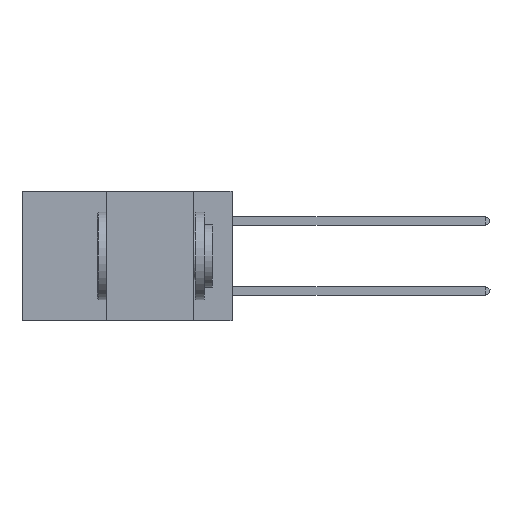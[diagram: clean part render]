
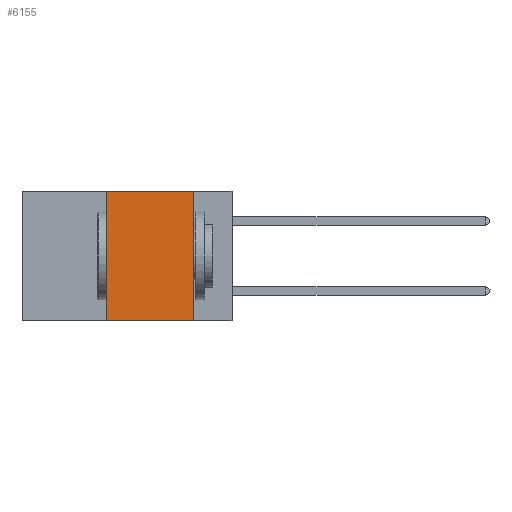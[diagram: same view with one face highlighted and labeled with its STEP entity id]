
A CAD part, left-side view. The second image highlights one B-rep face of the part: STEP entity #6155.
In plain terms, the highlighted planar face has unit normal (-1, 0, 0).
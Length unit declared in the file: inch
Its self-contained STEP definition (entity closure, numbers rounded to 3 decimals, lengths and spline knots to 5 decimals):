
#76 = VECTOR ( 'NONE', #8333, 39.37008 ) ;
#557 = DIRECTION ( 'NONE',  ( 0., 0., -1. ) ) ;
#728 = PLANE ( 'NONE',  #2168 ) ;
#819 = ORIENTED_EDGE ( 'NONE', *, *, #10191, .T. ) ;
#937 = ORIENTED_EDGE ( 'NONE', *, *, #7530, .F. ) ;
#1045 = VERTEX_POINT ( 'NONE', #1852 ) ;
#1852 = CARTESIAN_POINT ( 'NONE',  ( 0., 0.11, -0.37 ) ) ;
#2168 = AXIS2_PLACEMENT_3D ( 'NONE', #7407, #4162, #9220 ) ;
#2576 = CARTESIAN_POINT ( 'NONE',  ( 0., 0.36, 0. ) ) ;
#2775 = ORIENTED_EDGE ( 'NONE', *, *, #5032, .F. ) ;
#3537 = VECTOR ( 'NONE', #10254, 39.37008 ) ;
#3805 = VERTEX_POINT ( 'NONE', #9456 ) ;
#4162 = DIRECTION ( 'NONE',  ( 1., 0., 0. ) ) ;
#4769 = LINE ( 'NONE', #5936, #3537 ) ;
#5032 = EDGE_CURVE ( 'NONE', #3805, #1045, #9554, .T. ) ;
#5721 = LINE ( 'NONE', #2576, #6794 ) ;
#5936 = CARTESIAN_POINT ( 'NONE',  ( 0., 0.6, 0. ) ) ;
#6155 = ADVANCED_FACE ( 'NONE', ( #6179 ), #728, .F. ) ;
#6179 = FACE_OUTER_BOUND ( 'NONE', #7899, .T. ) ;
#6322 = CARTESIAN_POINT ( 'NONE',  ( 0., 0.36, 0. ) ) ;
#6646 = CARTESIAN_POINT ( 'NONE',  ( 0., 0.6, -0.37 ) ) ;
#6791 = VERTEX_POINT ( 'NONE', #9155 ) ;
#6794 = VECTOR ( 'NONE', #7733, 39.37008 ) ;
#7407 = CARTESIAN_POINT ( 'NONE',  ( 0., 0.6, 0. ) ) ;
#7530 = EDGE_CURVE ( 'NONE', #6791, #8830, #5721, .T. ) ;
#7684 = LINE ( 'NONE', #6646, #76 ) ;
#7733 = DIRECTION ( 'NONE',  ( 0., 0., 1. ) ) ;
#7734 = ORIENTED_EDGE ( 'NONE', *, *, #8209, .F. ) ;
#7899 = EDGE_LOOP ( 'NONE', ( #2775, #7734, #937, #819 ) ) ;
#8209 = EDGE_CURVE ( 'NONE', #8830, #3805, #4769, .T. ) ;
#8333 = DIRECTION ( 'NONE',  ( 0., -1., 0. ) ) ;
#8830 = VERTEX_POINT ( 'NONE', #6322 ) ;
#9155 = CARTESIAN_POINT ( 'NONE',  ( 0., 0.36, -0.37 ) ) ;
#9220 = DIRECTION ( 'NONE',  ( 0., 0., -1. ) ) ;
#9456 = CARTESIAN_POINT ( 'NONE',  ( 0., 0.11, 0. ) ) ;
#9554 = LINE ( 'NONE', #10596, #10213 ) ;
#10191 = EDGE_CURVE ( 'NONE', #6791, #1045, #7684, .T. ) ;
#10213 = VECTOR ( 'NONE', #557, 39.37008 ) ;
#10254 = DIRECTION ( 'NONE',  ( 0., -1., 0. ) ) ;
#10596 = CARTESIAN_POINT ( 'NONE',  ( 0., 0.11, 0. ) ) ;
